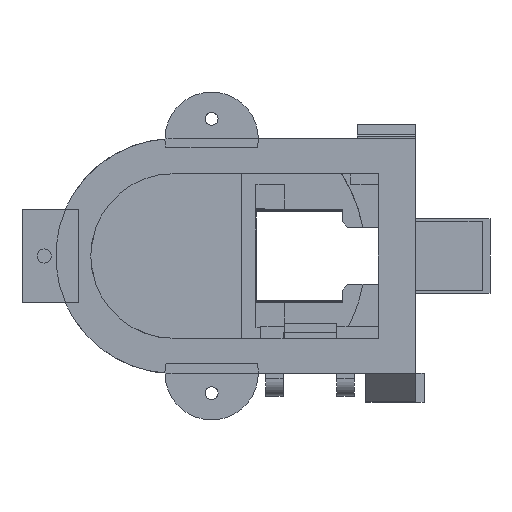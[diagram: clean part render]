
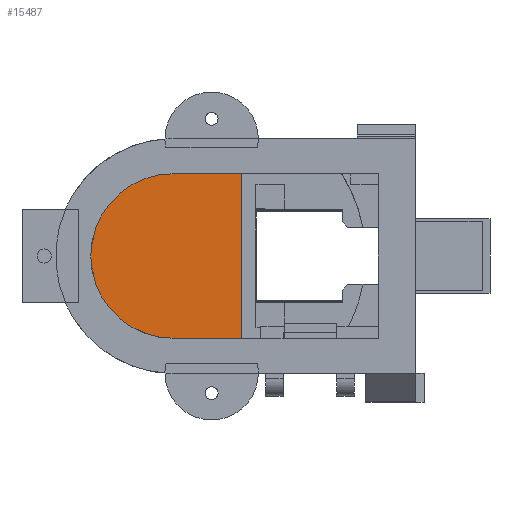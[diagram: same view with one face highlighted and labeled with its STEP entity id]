
A CAD part, left-side view. The second image highlights one B-rep face of the part: STEP entity #15487.
In plain terms, the highlighted planar face has unit normal (-1, 0, 0).
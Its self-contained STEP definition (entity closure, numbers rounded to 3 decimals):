
#2554 = CYLINDRICAL_SURFACE('',#2555,14.1);
#2555 = AXIS2_PLACEMENT_3D('',#2556,#2557,#2558);
#2556 = CARTESIAN_POINT('',(-19.05,47.913,0.));
#2557 = DIRECTION('',(1.,0.,0.));
#2558 = DIRECTION('',(0.,-1.,0.));
#2581 = PLANE('',#2582);
#2582 = AXIS2_PLACEMENT_3D('',#2583,#2584,#2585);
#2583 = CARTESIAN_POINT('',(-19.05,47.913,14.1));
#2584 = DIRECTION('',(0.,0.,1.));
#2585 = DIRECTION('',(0.,-1.,0.));
#2735 = PLANE('',#2736);
#2736 = AXIS2_PLACEMENT_3D('',#2737,#2738,#2739);
#2737 = CARTESIAN_POINT('',(-19.05,6.363,-14.1));
#2738 = DIRECTION('',(0.,0.,-1.));
#2739 = DIRECTION('',(0.,1.,0.));
#6885 = VERTEX_POINT('',#6886);
#6886 = CARTESIAN_POINT('',(-19.05,47.913,14.1));
#6907 = EDGE_CURVE('',#6885,#6908,#6910,.T.);
#6908 = VERTEX_POINT('',#6909);
#6909 = CARTESIAN_POINT('',(-19.05,47.913,-14.1));
#6910 = SURFACE_CURVE('',#6911,(#6916,#6923),.PCURVE_S1.);
#6911 = CIRCLE('',#6912,14.1);
#6912 = AXIS2_PLACEMENT_3D('',#6913,#6914,#6915);
#6913 = CARTESIAN_POINT('',(-19.05,47.913,0.));
#6914 = DIRECTION('',(-1.,0.,0.));
#6915 = DIRECTION('',(0.,-1.,0.));
#6916 = PCURVE('',#2554,#6917);
#6917 = DEFINITIONAL_REPRESENTATION('',(#6918),#6922);
#6918 = LINE('',#6919,#6920);
#6919 = CARTESIAN_POINT('',(6.283,0.));
#6920 = VECTOR('',#6921,1.);
#6921 = DIRECTION('',(-1.,0.));
#6922 = ( GEOMETRIC_REPRESENTATION_CONTEXT(2) 
PARAMETRIC_REPRESENTATION_CONTEXT() REPRESENTATION_CONTEXT('2D SPACE',''
  ) );
#6923 = PCURVE('',#6924,#6929);
#6924 = PLANE('',#6925);
#6925 = AXIS2_PLACEMENT_3D('',#6926,#6927,#6928);
#6926 = CARTESIAN_POINT('',(-19.05,13.081,-15.431));
#6927 = DIRECTION('',(-1.,0.,0.));
#6928 = DIRECTION('',(0.,0.,-1.));
#6929 = DEFINITIONAL_REPRESENTATION('',(#6930),#6934);
#6930 = CIRCLE('',#6931,14.1);
#6931 = AXIS2_PLACEMENT_2D('',#6932,#6933);
#6932 = CARTESIAN_POINT('',(-15.431,-34.832));
#6933 = DIRECTION('',(0.,1.));
#6934 = ( GEOMETRIC_REPRESENTATION_CONTEXT(2) 
PARAMETRIC_REPRESENTATION_CONTEXT() REPRESENTATION_CONTEXT('2D SPACE',''
  ) );
#9021 = EDGE_CURVE('',#9022,#6908,#9024,.T.);
#9022 = VERTEX_POINT('',#9023);
#9023 = CARTESIAN_POINT('',(-19.05,36.099,-14.1));
#9024 = SURFACE_CURVE('',#9025,(#9029,#9036),.PCURVE_S1.);
#9025 = LINE('',#9026,#9027);
#9026 = CARTESIAN_POINT('',(-19.05,6.363,-14.1));
#9027 = VECTOR('',#9028,1.);
#9028 = DIRECTION('',(0.,1.,0.));
#9029 = PCURVE('',#2735,#9030);
#9030 = DEFINITIONAL_REPRESENTATION('',(#9031),#9035);
#9031 = LINE('',#9032,#9033);
#9032 = CARTESIAN_POINT('',(0.,0.));
#9033 = VECTOR('',#9034,1.);
#9034 = DIRECTION('',(1.,0.));
#9035 = ( GEOMETRIC_REPRESENTATION_CONTEXT(2) 
PARAMETRIC_REPRESENTATION_CONTEXT() REPRESENTATION_CONTEXT('2D SPACE',''
  ) );
#9036 = PCURVE('',#6924,#9037);
#9037 = DEFINITIONAL_REPRESENTATION('',(#9038),#9042);
#9038 = LINE('',#9039,#9040);
#9039 = CARTESIAN_POINT('',(-1.331,6.718));
#9040 = VECTOR('',#9041,1.);
#9041 = DIRECTION('',(0.,-1.));
#9042 = ( GEOMETRIC_REPRESENTATION_CONTEXT(2) 
PARAMETRIC_REPRESENTATION_CONTEXT() REPRESENTATION_CONTEXT('2D SPACE',''
  ) );
#9073 = EDGE_CURVE('',#6885,#9074,#9076,.T.);
#9074 = VERTEX_POINT('',#9075);
#9075 = CARTESIAN_POINT('',(-19.05,36.099,14.1));
#9076 = SURFACE_CURVE('',#9077,(#9081,#9088),.PCURVE_S1.);
#9077 = LINE('',#9078,#9079);
#9078 = CARTESIAN_POINT('',(-19.05,47.913,14.1));
#9079 = VECTOR('',#9080,1.);
#9080 = DIRECTION('',(0.,-1.,0.));
#9081 = PCURVE('',#2581,#9082);
#9082 = DEFINITIONAL_REPRESENTATION('',(#9083),#9087);
#9083 = LINE('',#9084,#9085);
#9084 = CARTESIAN_POINT('',(0.,0.));
#9085 = VECTOR('',#9086,1.);
#9086 = DIRECTION('',(1.,0.));
#9087 = ( GEOMETRIC_REPRESENTATION_CONTEXT(2) 
PARAMETRIC_REPRESENTATION_CONTEXT() REPRESENTATION_CONTEXT('2D SPACE',''
  ) );
#9088 = PCURVE('',#6924,#9089);
#9089 = DEFINITIONAL_REPRESENTATION('',(#9090),#9094);
#9090 = LINE('',#9091,#9092);
#9091 = CARTESIAN_POINT('',(-29.531,-34.832));
#9092 = VECTOR('',#9093,1.);
#9093 = DIRECTION('',(0.,1.));
#9094 = ( GEOMETRIC_REPRESENTATION_CONTEXT(2) 
PARAMETRIC_REPRESENTATION_CONTEXT() REPRESENTATION_CONTEXT('2D SPACE',''
  ) );
#15487 = ADVANCED_FACE('',(#15488),#6924,.T.);
#15488 = FACE_BOUND('',#15489,.T.);
#15489 = EDGE_LOOP('',(#15490,#15491,#15517,#15518));
#15490 = ORIENTED_EDGE('',*,*,#9021,.F.);
#15491 = ORIENTED_EDGE('',*,*,#15492,.F.);
#15492 = EDGE_CURVE('',#9074,#9022,#15493,.T.);
#15493 = SURFACE_CURVE('',#15494,(#15498,#15505),.PCURVE_S1.);
#15494 = LINE('',#15495,#15496);
#15495 = CARTESIAN_POINT('',(-19.05,36.099,14.667));
#15496 = VECTOR('',#15497,1.);
#15497 = DIRECTION('',(0.,0.,-1.));
#15498 = PCURVE('',#6924,#15499);
#15499 = DEFINITIONAL_REPRESENTATION('',(#15500),#15504);
#15500 = LINE('',#15501,#15502);
#15501 = CARTESIAN_POINT('',(-30.098,-23.018));
#15502 = VECTOR('',#15503,1.);
#15503 = DIRECTION('',(1.,0.));
#15504 = ( GEOMETRIC_REPRESENTATION_CONTEXT(2) 
PARAMETRIC_REPRESENTATION_CONTEXT() REPRESENTATION_CONTEXT('2D SPACE',''
  ) );
#15505 = PCURVE('',#15506,#15511);
#15506 = PLANE('',#15507);
#15507 = AXIS2_PLACEMENT_3D('',#15508,#15509,#15510);
#15508 = CARTESIAN_POINT('',(-19.05,36.099,14.667));
#15509 = DIRECTION('',(0.,1.,0.));
#15510 = DIRECTION('',(0.,0.,-1.));
#15511 = DEFINITIONAL_REPRESENTATION('',(#15512),#15516);
#15512 = LINE('',#15513,#15514);
#15513 = CARTESIAN_POINT('',(0.,0.));
#15514 = VECTOR('',#15515,1.);
#15515 = DIRECTION('',(1.,0.));
#15516 = ( GEOMETRIC_REPRESENTATION_CONTEXT(2) 
PARAMETRIC_REPRESENTATION_CONTEXT() REPRESENTATION_CONTEXT('2D SPACE',''
  ) );
#15517 = ORIENTED_EDGE('',*,*,#9073,.F.);
#15518 = ORIENTED_EDGE('',*,*,#6907,.T.);
